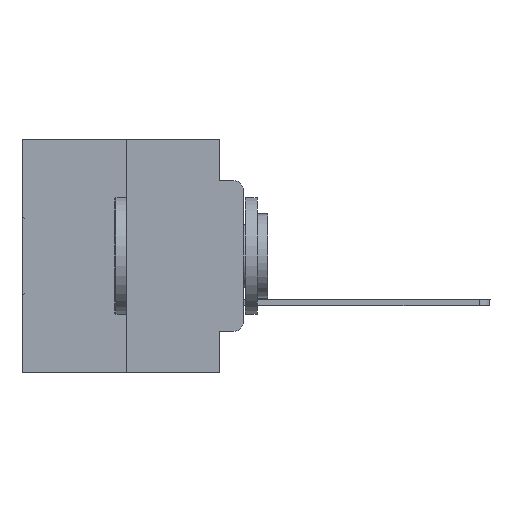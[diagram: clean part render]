
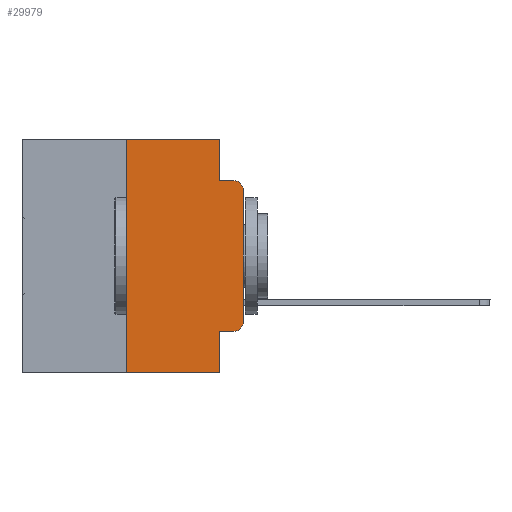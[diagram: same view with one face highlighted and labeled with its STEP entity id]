
A CAD part, left-side view. The second image highlights one B-rep face of the part: STEP entity #29979.
In plain terms, the highlighted planar face has unit normal (-1, 0, 0).
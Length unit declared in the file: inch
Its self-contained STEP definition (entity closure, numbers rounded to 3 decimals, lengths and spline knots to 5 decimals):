
#491 = ORIENTED_EDGE ( 'NONE', *, *, #28207, .T. ) ;
#669 = CARTESIAN_POINT ( 'NONE',  ( 0., 0., -0.3915 ) ) ;
#815 = CARTESIAN_POINT ( 'NONE',  ( 0., 0.473, 0. ) ) ;
#1244 = AXIS2_PLACEMENT_3D ( 'NONE', #12288, #9655, #19733 ) ;
#1292 = ORIENTED_EDGE ( 'NONE', *, *, #1473, .T. ) ;
#1433 = DIRECTION ( 'NONE',  ( 0., 0., 1. ) ) ;
#1473 = EDGE_CURVE ( 'NONE', #4632, #14837, #28130, .T. ) ;
#1595 = DIRECTION ( 'NONE',  ( 0., -1., 0. ) ) ;
#1758 = CARTESIAN_POINT ( 'NONE',  ( 0., 0.473, 0. ) ) ;
#2308 = CARTESIAN_POINT ( 'NONE',  ( 0., 0.051, 0. ) ) ;
#2857 = EDGE_LOOP ( 'NONE', ( #12012, #491, #26009, #30513, #16258, #28498, #31267, #28879, #28171, #1292 ) ) ;
#3221 = CARTESIAN_POINT ( 'NONE',  ( 0., 0.051, -0.4115 ) ) ;
#3463 = FACE_OUTER_BOUND ( 'NONE', #2857, .T. ) ;
#4088 = CIRCLE ( 'NONE', #30457, 0.02 ) ;
#4632 = VERTEX_POINT ( 'NONE', #9125 ) ;
#5820 = DIRECTION ( 'NONE',  ( -1., 0., 0. ) ) ;
#8127 = VERTEX_POINT ( 'NONE', #3221 ) ;
#8668 = VERTEX_POINT ( 'NONE', #18168 ) ;
#8669 = LINE ( 'NONE', #29149, #13617 ) ;
#8940 = DIRECTION ( 'NONE',  ( 0., -1., 0. ) ) ;
#9125 = CARTESIAN_POINT ( 'NONE',  ( 0., 0.02, -0.4115 ) ) ;
#9282 = VERTEX_POINT ( 'NONE', #30946 ) ;
#9383 = CARTESIAN_POINT ( 'NONE',  ( 0., 0.02, -0.0885 ) ) ;
#9655 = DIRECTION ( 'NONE',  ( -1., 0., 0. ) ) ;
#10739 = VERTEX_POINT ( 'NONE', #21589 ) ;
#11043 = CARTESIAN_POINT ( 'NONE',  ( 0., 0.051, 0. ) ) ;
#11798 = EDGE_CURVE ( 'NONE', #8127, #4632, #26670, .T. ) ;
#11847 = CARTESIAN_POINT ( 'NONE',  ( 0., 0.051, 0. ) ) ;
#11895 = VECTOR ( 'NONE', #8940, 39.37008 ) ;
#12012 = ORIENTED_EDGE ( 'NONE', *, *, #30371, .T. ) ;
#12211 = DIRECTION ( 'NONE',  ( 0., 0., -1. ) ) ;
#12288 = CARTESIAN_POINT ( 'NONE',  ( 0., 0.02, -0.3915 ) ) ;
#13617 = VECTOR ( 'NONE', #1433, 39.37008 ) ;
#14732 = AXIS2_PLACEMENT_3D ( 'NONE', #815, #21458, #26255 ) ;
#14837 = VERTEX_POINT ( 'NONE', #669 ) ;
#14843 = DIRECTION ( 'NONE',  ( 0., -1., 0. ) ) ;
#15107 = VECTOR ( 'NONE', #16938, 39.37008 ) ;
#16258 = ORIENTED_EDGE ( 'NONE', *, *, #25947, .F. ) ;
#16607 = LINE ( 'NONE', #1758, #15107 ) ;
#16938 = DIRECTION ( 'NONE',  ( 0., -1., 0. ) ) ;
#17274 = VECTOR ( 'NONE', #14843, 39.37008 ) ;
#17640 = LINE ( 'NONE', #2308, #32562 ) ;
#18168 = CARTESIAN_POINT ( 'NONE',  ( 0., 0.25, -0.5 ) ) ;
#18239 = EDGE_CURVE ( 'NONE', #19246, #24329, #32349, .T. ) ;
#18363 = CARTESIAN_POINT ( 'NONE',  ( 0., 0.02, -0.1085 ) ) ;
#18509 = CARTESIAN_POINT ( 'NONE',  ( 0., 0.051, -0.0885 ) ) ;
#19028 = CARTESIAN_POINT ( 'NONE',  ( 0., 0.473, -0.5 ) ) ;
#19246 = VERTEX_POINT ( 'NONE', #18509 ) ;
#19733 = DIRECTION ( 'NONE',  ( 0., 0., -1. ) ) ;
#20718 = CARTESIAN_POINT ( 'NONE',  ( 0., 0., -0.1085 ) ) ;
#21247 = LINE ( 'NONE', #28358, #27174 ) ;
#21458 = DIRECTION ( 'NONE',  ( 1., 0., 0. ) ) ;
#21589 = CARTESIAN_POINT ( 'NONE',  ( 0., 0.051, -0.5 ) ) ;
#21937 = LINE ( 'NONE', #11847, #24075 ) ;
#22514 = EDGE_CURVE ( 'NONE', #28615, #19246, #17640, .T. ) ;
#23291 = EDGE_CURVE ( 'NONE', #8668, #9282, #8669, .T. ) ;
#24075 = VECTOR ( 'NONE', #29537, 39.37008 ) ;
#24329 = VERTEX_POINT ( 'NONE', #9383 ) ;
#25015 = EDGE_CURVE ( 'NONE', #8668, #10739, #31396, .T. ) ;
#25530 = EDGE_CURVE ( 'NONE', #8127, #10739, #21937, .T. ) ;
#25947 = EDGE_CURVE ( 'NONE', #9282, #28615, #16607, .T. ) ;
#26009 = ORIENTED_EDGE ( 'NONE', *, *, #18239, .F. ) ;
#26237 = VERTEX_POINT ( 'NONE', #20718 ) ;
#26255 = DIRECTION ( 'NONE',  ( 0., 0., -1. ) ) ;
#26522 = DIRECTION ( 'NONE',  ( 0., 0., 1. ) ) ;
#26558 = PLANE ( 'NONE',  #14732 ) ;
#26670 = LINE ( 'NONE', #26844, #32162 ) ;
#26844 = CARTESIAN_POINT ( 'NONE',  ( 0., 0.051, -0.4115 ) ) ;
#27053 = CARTESIAN_POINT ( 'NONE',  ( 0., 0.051, -0.0885 ) ) ;
#27174 = VECTOR ( 'NONE', #26522, 39.37008 ) ;
#28130 = CIRCLE ( 'NONE', #1244, 0.02 ) ;
#28171 = ORIENTED_EDGE ( 'NONE', *, *, #11798, .T. ) ;
#28207 = EDGE_CURVE ( 'NONE', #26237, #24329, #4088, .T. ) ;
#28358 = CARTESIAN_POINT ( 'NONE',  ( 0., 0., 0. ) ) ;
#28440 = DIRECTION ( 'NONE',  ( 0., 0., -1. ) ) ;
#28498 = ORIENTED_EDGE ( 'NONE', *, *, #23291, .F. ) ;
#28615 = VERTEX_POINT ( 'NONE', #11043 ) ;
#28879 = ORIENTED_EDGE ( 'NONE', *, *, #25530, .F. ) ;
#29149 = CARTESIAN_POINT ( 'NONE',  ( 0., 0.25, 0. ) ) ;
#29537 = DIRECTION ( 'NONE',  ( 0., 0., -1. ) ) ;
#29979 = ADVANCED_FACE ( 'NONE', ( #3463 ), #26558, .F. ) ;
#30371 = EDGE_CURVE ( 'NONE', #14837, #26237, #21247, .T. ) ;
#30457 = AXIS2_PLACEMENT_3D ( 'NONE', #18363, #5820, #28440 ) ;
#30513 = ORIENTED_EDGE ( 'NONE', *, *, #22514, .F. ) ;
#30946 = CARTESIAN_POINT ( 'NONE',  ( 0., 0.25, 0. ) ) ;
#31267 = ORIENTED_EDGE ( 'NONE', *, *, #25015, .T. ) ;
#31396 = LINE ( 'NONE', #19028, #11895 ) ;
#32162 = VECTOR ( 'NONE', #1595, 39.37008 ) ;
#32349 = LINE ( 'NONE', #27053, #17274 ) ;
#32562 = VECTOR ( 'NONE', #12211, 39.37008 ) ;
